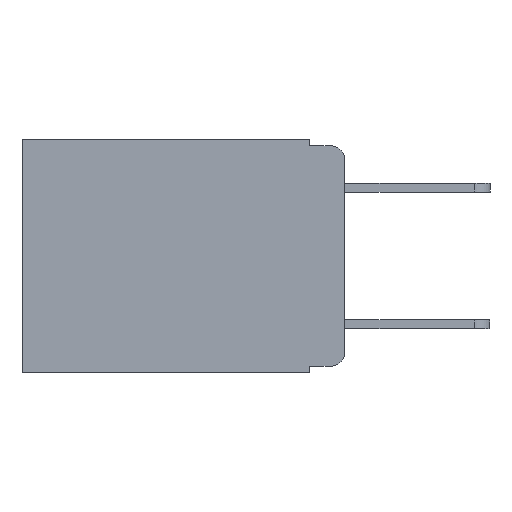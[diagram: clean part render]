
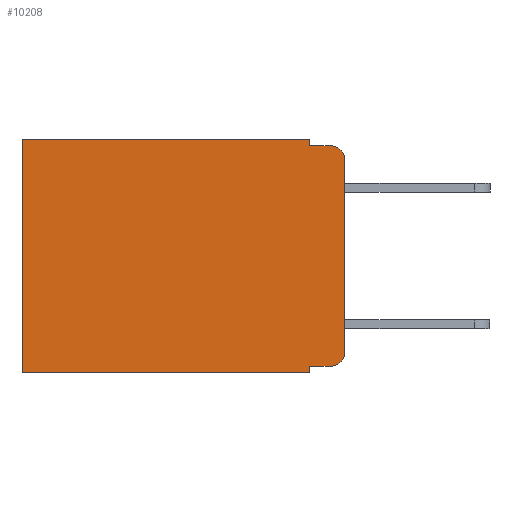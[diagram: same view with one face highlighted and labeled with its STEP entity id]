
A CAD part, left-side view. The second image highlights one B-rep face of the part: STEP entity #10208.
In plain terms, the highlighted planar face has unit normal (-1, 0, 0).
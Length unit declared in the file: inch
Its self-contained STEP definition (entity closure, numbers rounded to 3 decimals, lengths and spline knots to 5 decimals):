
#6 = VERTEX_POINT ( 'NONE', #2432 ) ;
#292 = VERTEX_POINT ( 'NONE', #321 ) ;
#321 = CARTESIAN_POINT ( 'NONE',  ( 0.298, 0.051, 0. ) ) ;
#346 = VECTOR ( 'NONE', #16622, 39.37008 ) ;
#366 = CARTESIAN_POINT ( 'NONE',  ( 0.298, 0.051, -0.333 ) ) ;
#1393 = DIRECTION ( 'NONE',  ( 0., -1., 0. ) ) ;
#1575 = LINE ( 'NONE', #9866, #15595 ) ;
#1746 = CARTESIAN_POINT ( 'NONE',  ( 0.298, 0., -0.03 ) ) ;
#2053 = VECTOR ( 'NONE', #8014, 39.37008 ) ;
#2432 = CARTESIAN_POINT ( 'NONE',  ( 0.298, 0.473, 0. ) ) ;
#2441 = AXIS2_PLACEMENT_3D ( 'NONE', #4997, #17101, #6771 ) ;
#2549 = AXIS2_PLACEMENT_3D ( 'NONE', #5886, #11069, #6919 ) ;
#2802 = DIRECTION ( 'NONE',  ( 0., 0., -1. ) ) ;
#2826 = DIRECTION ( 'NONE',  ( 0., 1., 0. ) ) ;
#2871 = ORIENTED_EDGE ( 'NONE', *, *, #6522, .F. ) ;
#2886 = VECTOR ( 'NONE', #13084, 39.37008 ) ;
#2960 = EDGE_CURVE ( 'NONE', #6449, #12021, #12376, .T. ) ;
#3619 = VERTEX_POINT ( 'NONE', #12902 ) ;
#3662 = VECTOR ( 'NONE', #2802, 39.37008 ) ;
#3684 = ORIENTED_EDGE ( 'NONE', *, *, #14353, .T. ) ;
#3758 = VERTEX_POINT ( 'NONE', #6548 ) ;
#3980 = VERTEX_POINT ( 'NONE', #366 ) ;
#4412 = VERTEX_POINT ( 'NONE', #12159 ) ;
#4972 = CARTESIAN_POINT ( 'NONE',  ( 0.298, 0.051, -0.01 ) ) ;
#4997 = CARTESIAN_POINT ( 'NONE',  ( 0.298, 0., 0. ) ) ;
#5232 = LINE ( 'NONE', #9712, #346 ) ;
#5696 = VERTEX_POINT ( 'NONE', #10794 ) ;
#5886 = CARTESIAN_POINT ( 'NONE',  ( 0.298, 0.02, -0.313 ) ) ;
#5916 = VERTEX_POINT ( 'NONE', #11621 ) ;
#6029 = DIRECTION ( 'NONE',  ( -1., 0., 0. ) ) ;
#6449 = VERTEX_POINT ( 'NONE', #1746 ) ;
#6522 = EDGE_CURVE ( 'NONE', #292, #3758, #13098, .T. ) ;
#6548 = CARTESIAN_POINT ( 'NONE',  ( 0.298, 0.051, -0.01 ) ) ;
#6771 = DIRECTION ( 'NONE',  ( 0., 0., -1. ) ) ;
#6811 = EDGE_CURVE ( 'NONE', #5916, #3619, #7605, .T. ) ;
#6919 = DIRECTION ( 'NONE',  ( 0., 0., -1. ) ) ;
#7233 = EDGE_CURVE ( 'NONE', #3980, #5696, #8139, .T. ) ;
#7451 = ORIENTED_EDGE ( 'NONE', *, *, #17243, .T. ) ;
#7466 = DIRECTION ( 'NONE',  ( 0., 0., -1. ) ) ;
#7605 = CIRCLE ( 'NONE', #2549, 0.02 ) ;
#7758 = ORIENTED_EDGE ( 'NONE', *, *, #8865, .F. ) ;
#8014 = DIRECTION ( 'NONE',  ( 0., 0., -1. ) ) ;
#8139 = LINE ( 'NONE', #15715, #2886 ) ;
#8863 = ORIENTED_EDGE ( 'NONE', *, *, #13100, .T. ) ;
#8865 = EDGE_CURVE ( 'NONE', #3758, #12021, #9434, .T. ) ;
#9434 = LINE ( 'NONE', #4972, #21895 ) ;
#9712 = CARTESIAN_POINT ( 'NONE',  ( 0.298, 0.051, -0.333 ) ) ;
#9866 = CARTESIAN_POINT ( 'NONE',  ( 0.298, 0., 0. ) ) ;
#9940 = ORIENTED_EDGE ( 'NONE', *, *, #7233, .F. ) ;
#10092 = ORIENTED_EDGE ( 'NONE', *, *, #19619, .F. ) ;
#10208 = ADVANCED_FACE ( 'NONE', ( #12333 ), #13703, .F. ) ;
#10660 = AXIS2_PLACEMENT_3D ( 'NONE', #14841, #6029, #16386 ) ;
#10794 = CARTESIAN_POINT ( 'NONE',  ( 0.298, 0.051, -0.343 ) ) ;
#11039 = ORIENTED_EDGE ( 'NONE', *, *, #6811, .T. ) ;
#11069 = DIRECTION ( 'NONE',  ( -1., 0., 0. ) ) ;
#11621 = CARTESIAN_POINT ( 'NONE',  ( 0.298, 0.02, -0.333 ) ) ;
#12021 = VERTEX_POINT ( 'NONE', #21941 ) ;
#12050 = LINE ( 'NONE', #18298, #2053 ) ;
#12159 = CARTESIAN_POINT ( 'NONE',  ( 0.298, 0.473, -0.343 ) ) ;
#12333 = FACE_OUTER_BOUND ( 'NONE', #18709, .T. ) ;
#12376 = CIRCLE ( 'NONE', #10660, 0.02 ) ;
#12902 = CARTESIAN_POINT ( 'NONE',  ( 0.298, 0., -0.313 ) ) ;
#13084 = DIRECTION ( 'NONE',  ( 0., 0., -1. ) ) ;
#13098 = LINE ( 'NONE', #16275, #22012 ) ;
#13100 = EDGE_CURVE ( 'NONE', #6, #4412, #17474, .T. ) ;
#13703 = PLANE ( 'NONE',  #2441 ) ;
#13819 = CARTESIAN_POINT ( 'NONE',  ( 0.298, 0., -0.343 ) ) ;
#14353 = EDGE_CURVE ( 'NONE', #292, #6, #1575, .T. ) ;
#14841 = CARTESIAN_POINT ( 'NONE',  ( 0.298, 0.02, -0.03 ) ) ;
#15595 = VECTOR ( 'NONE', #2826, 39.37008 ) ;
#15687 = LINE ( 'NONE', #13819, #19627 ) ;
#15715 = CARTESIAN_POINT ( 'NONE',  ( 0.298, 0.051, 0. ) ) ;
#16275 = CARTESIAN_POINT ( 'NONE',  ( 0.298, 0.051, 0. ) ) ;
#16386 = DIRECTION ( 'NONE',  ( 0., 0., -1. ) ) ;
#16622 = DIRECTION ( 'NONE',  ( 0., -1., 0. ) ) ;
#17101 = DIRECTION ( 'NONE',  ( 1., 0., 0. ) ) ;
#17243 = EDGE_CURVE ( 'NONE', #3980, #5916, #5232, .T. ) ;
#17398 = ORIENTED_EDGE ( 'NONE', *, *, #21117, .F. ) ;
#17474 = LINE ( 'NONE', #21689, #3662 ) ;
#17731 = ORIENTED_EDGE ( 'NONE', *, *, #2960, .T. ) ;
#18298 = CARTESIAN_POINT ( 'NONE',  ( 0.298, 0., 0. ) ) ;
#18709 = EDGE_LOOP ( 'NONE', ( #10092, #17731, #7758, #2871, #3684, #8863, #17398, #9940, #7451, #11039 ) ) ;
#18899 = DIRECTION ( 'NONE',  ( 0., 1., 0. ) ) ;
#19619 = EDGE_CURVE ( 'NONE', #6449, #3619, #12050, .T. ) ;
#19627 = VECTOR ( 'NONE', #18899, 39.37008 ) ;
#21117 = EDGE_CURVE ( 'NONE', #5696, #4412, #15687, .T. ) ;
#21689 = CARTESIAN_POINT ( 'NONE',  ( 0.298, 0.473, 0. ) ) ;
#21895 = VECTOR ( 'NONE', #1393, 39.37008 ) ;
#21941 = CARTESIAN_POINT ( 'NONE',  ( 0.298, 0.02, -0.01 ) ) ;
#22012 = VECTOR ( 'NONE', #7466, 39.37008 ) ;
